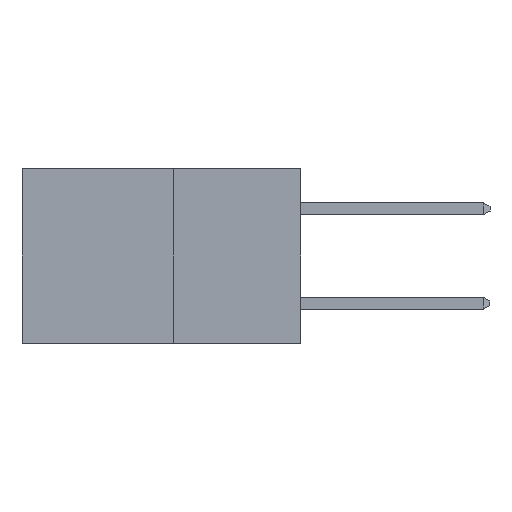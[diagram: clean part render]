
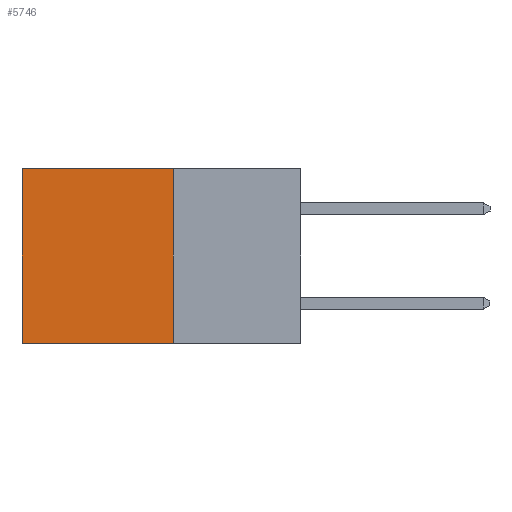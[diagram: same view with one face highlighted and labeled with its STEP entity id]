
A CAD part, left-side view. The second image highlights one B-rep face of the part: STEP entity #5746.
In plain terms, the highlighted planar face has unit normal (-1, 0, 0).
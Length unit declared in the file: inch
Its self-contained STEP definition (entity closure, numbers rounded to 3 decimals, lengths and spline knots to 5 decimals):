
#225 = FACE_OUTER_BOUND ( 'NONE', #6858, .T. ) ;
#241 = CARTESIAN_POINT ( 'NONE',  ( 0.277, 0.59, -0.37 ) ) ;
#335 = DIRECTION ( 'NONE',  ( 1., 0., 0. ) ) ;
#344 = CARTESIAN_POINT ( 'NONE',  ( 0.277, 0.27, -0.37 ) ) ;
#383 = VERTEX_POINT ( 'NONE', #5951 ) ;
#387 = EDGE_CURVE ( 'NONE', #5498, #6336, #675, .T. ) ;
#554 = AXIS2_PLACEMENT_3D ( 'NONE', #344, #335, #605 ) ;
#605 = DIRECTION ( 'NONE',  ( 0., 0., -1. ) ) ;
#675 = LINE ( 'NONE', #1089, #7002 ) ;
#1089 = CARTESIAN_POINT ( 'NONE',  ( 0.277, 0.27, -0.37 ) ) ;
#1604 = EDGE_CURVE ( 'NONE', #5498, #383, #6688, .T. ) ;
#1668 = ORIENTED_EDGE ( 'NONE', *, *, #4194, .F. ) ;
#1831 = CARTESIAN_POINT ( 'NONE',  ( 0.277, 0.27, 0. ) ) ;
#2263 = CARTESIAN_POINT ( 'NONE',  ( 0.277, 0.27, -0.37 ) ) ;
#2366 = DIRECTION ( 'NONE',  ( 0., 1., 0. ) ) ;
#2698 = VECTOR ( 'NONE', #2366, 39.37008 ) ;
#2798 = VECTOR ( 'NONE', #5620, 39.37008 ) ;
#2834 = EDGE_CURVE ( 'NONE', #383, #2956, #4444, .T. ) ;
#2956 = VERTEX_POINT ( 'NONE', #241 ) ;
#3119 = ORIENTED_EDGE ( 'NONE', *, *, #1604, .T. ) ;
#3653 = CARTESIAN_POINT ( 'NONE',  ( 0.277, 0.27, 0. ) ) ;
#3786 = CARTESIAN_POINT ( 'NONE',  ( 0.277, 0.27, -0.37 ) ) ;
#3900 = VECTOR ( 'NONE', #7156, 39.37008 ) ;
#4194 = EDGE_CURVE ( 'NONE', #6336, #2956, #4344, .T. ) ;
#4344 = LINE ( 'NONE', #2263, #2698 ) ;
#4382 = DIRECTION ( 'NONE',  ( 0., 0., -1. ) ) ;
#4444 = LINE ( 'NONE', #5713, #2798 ) ;
#5498 = VERTEX_POINT ( 'NONE', #1831 ) ;
#5620 = DIRECTION ( 'NONE',  ( 0., 0., -1. ) ) ;
#5713 = CARTESIAN_POINT ( 'NONE',  ( 0.277, 0.59, -0.37 ) ) ;
#5746 = ADVANCED_FACE ( 'NONE', ( #225 ), #6712, .F. ) ;
#5951 = CARTESIAN_POINT ( 'NONE',  ( 0.277, 0.59, 0. ) ) ;
#6299 = ORIENTED_EDGE ( 'NONE', *, *, #387, .F. ) ;
#6336 = VERTEX_POINT ( 'NONE', #3786 ) ;
#6503 = ORIENTED_EDGE ( 'NONE', *, *, #2834, .T. ) ;
#6688 = LINE ( 'NONE', #3653, #3900 ) ;
#6712 = PLANE ( 'NONE',  #554 ) ;
#6858 = EDGE_LOOP ( 'NONE', ( #6503, #1668, #6299, #3119 ) ) ;
#7002 = VECTOR ( 'NONE', #4382, 39.37008 ) ;
#7156 = DIRECTION ( 'NONE',  ( 0., 1., 0. ) ) ;
